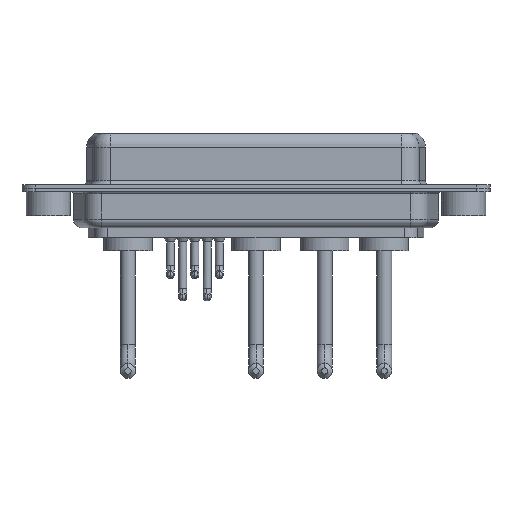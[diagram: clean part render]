
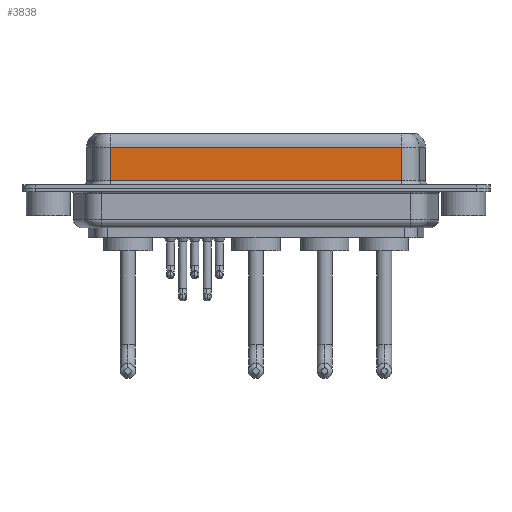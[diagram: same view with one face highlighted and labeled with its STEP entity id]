
A CAD part, front view. The second image highlights one B-rep face of the part: STEP entity #3838.
In plain terms, the highlighted planar face has unit normal (0, -1, 0).
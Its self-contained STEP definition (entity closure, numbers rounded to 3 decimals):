
#620 = CARTESIAN_POINT ( 'NONE',  ( 7.013, -3.95, 6.4 ) ) ;
#711 = CARTESIAN_POINT ( 'NONE',  ( 40.037, -3.95, 0.9 ) ) ;
#760 = ORIENTED_EDGE ( 'NONE', *, *, #15526, .T. ) ;
#809 = EDGE_CURVE ( 'NONE', #5147, #7606, #14879, .T. ) ;
#1003 = DIRECTION ( 'NONE',  ( 1., 0., 0. ) ) ;
#1130 = CARTESIAN_POINT ( 'NONE',  ( 40.037, -3.95, 4.65 ) ) ;
#3249 = VECTOR ( 'NONE', #15379, 1000. ) ;
#3605 = VECTOR ( 'NONE', #13601, 1000. ) ;
#3838 = ADVANCED_FACE ( 'NONE', ( #5890 ), #11211, .F. ) ;
#4408 = CARTESIAN_POINT ( 'NONE',  ( 7.013, -3.95, 4.65 ) ) ;
#4530 = DIRECTION ( 'NONE',  ( -1., 0., 0. ) ) ;
#4910 = VECTOR ( 'NONE', #1003, 1000. ) ;
#5147 = VERTEX_POINT ( 'NONE', #1130 ) ;
#5166 = ORIENTED_EDGE ( 'NONE', *, *, #809, .T. ) ;
#5890 = FACE_OUTER_BOUND ( 'NONE', #8753, .T. ) ;
#6871 = EDGE_CURVE ( 'NONE', #7606, #12949, #7230, .T. ) ;
#6917 = DIRECTION ( 'NONE',  ( 0., 0., 1. ) ) ;
#7230 = LINE ( 'NONE', #620, #3605 ) ;
#7606 = VERTEX_POINT ( 'NONE', #4408 ) ;
#8080 = VECTOR ( 'NONE', #4530, 1000. ) ;
#8279 = ORIENTED_EDGE ( 'NONE', *, *, #6871, .T. ) ;
#8520 = CARTESIAN_POINT ( 'NONE',  ( 7.013, -3.95, 0.9 ) ) ;
#8525 = CARTESIAN_POINT ( 'NONE',  ( 40.037, -3.95, 4.65 ) ) ;
#8753 = EDGE_LOOP ( 'NONE', ( #14613, #5166, #8279, #760 ) ) ;
#10326 = LINE ( 'NONE', #14244, #4910 ) ;
#10589 = VERTEX_POINT ( 'NONE', #711 ) ;
#11211 = PLANE ( 'NONE',  #12035 ) ;
#12035 = AXIS2_PLACEMENT_3D ( 'NONE', #14954, #13734, #6917 ) ;
#12949 = VERTEX_POINT ( 'NONE', #8520 ) ;
#13601 = DIRECTION ( 'NONE',  ( 0., 0., -1. ) ) ;
#13734 = DIRECTION ( 'NONE',  ( 0., 1., 0. ) ) ;
#14244 = CARTESIAN_POINT ( 'NONE',  ( 40.037, -3.95, 0.9 ) ) ;
#14613 = ORIENTED_EDGE ( 'NONE', *, *, #15385, .F. ) ;
#14879 = LINE ( 'NONE', #8525, #8080 ) ;
#14954 = CARTESIAN_POINT ( 'NONE',  ( 40.037, -3.95, 6.4 ) ) ;
#15211 = CARTESIAN_POINT ( 'NONE',  ( 40.037, -3.95, 6.4 ) ) ;
#15379 = DIRECTION ( 'NONE',  ( 0., 0., -1. ) ) ;
#15385 = EDGE_CURVE ( 'NONE', #5147, #10589, #16521, .T. ) ;
#15526 = EDGE_CURVE ( 'NONE', #12949, #10589, #10326, .T. ) ;
#16521 = LINE ( 'NONE', #15211, #3249 ) ;
